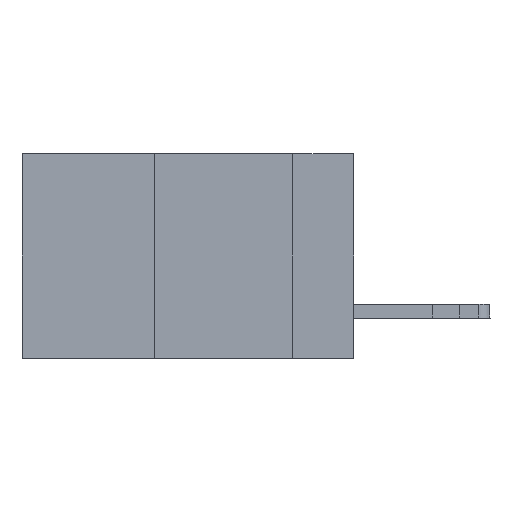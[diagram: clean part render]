
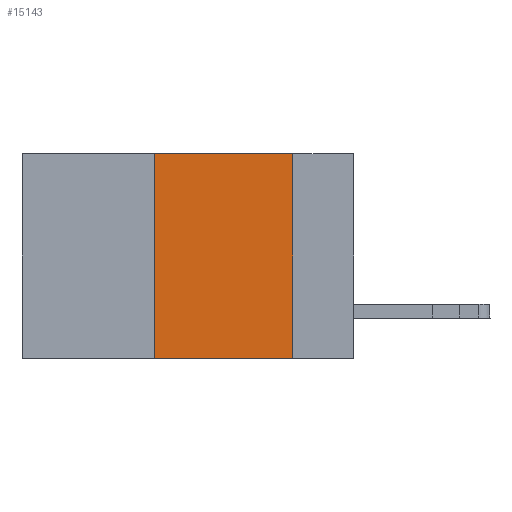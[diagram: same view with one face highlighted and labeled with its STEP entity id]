
A CAD part, left-side view. The second image highlights one B-rep face of the part: STEP entity #15143.
In plain terms, the highlighted planar face has unit normal (-1, 0, 0).
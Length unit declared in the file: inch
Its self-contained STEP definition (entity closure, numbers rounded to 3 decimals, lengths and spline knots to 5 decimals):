
#76 = DIRECTION ( 'NONE',  ( 0., -1., 0. ) ) ;
#1234 = ORIENTED_EDGE ( 'NONE', *, *, #23813, .F. ) ;
#3835 = CARTESIAN_POINT ( 'NONE',  ( 0., 0.6, 0. ) ) ;
#4667 = DIRECTION ( 'NONE',  ( 1., 0., 0. ) ) ;
#5010 = EDGE_CURVE ( 'NONE', #21064, #9253, #13825, .T. ) ;
#5304 = VERTEX_POINT ( 'NONE', #12621 ) ;
#5528 = LINE ( 'NONE', #25120, #19961 ) ;
#6491 = ORIENTED_EDGE ( 'NONE', *, *, #9548, .F. ) ;
#8597 = VECTOR ( 'NONE', #76, 39.37008 ) ;
#8794 = EDGE_LOOP ( 'NONE', ( #1234, #21076, #6491, #24580 ) ) ;
#9253 = VERTEX_POINT ( 'NONE', #19338 ) ;
#9548 = EDGE_CURVE ( 'NONE', #13042, #21064, #21270, .T. ) ;
#11204 = EDGE_CURVE ( 'NONE', #13042, #5304, #11600, .T. ) ;
#11600 = LINE ( 'NONE', #24869, #24228 ) ;
#12329 = CARTESIAN_POINT ( 'NONE',  ( 0., 0.36, 0. ) ) ;
#12369 = PLANE ( 'NONE',  #20666 ) ;
#12621 = CARTESIAN_POINT ( 'NONE',  ( 0., 0.11, -0.37 ) ) ;
#12717 = CARTESIAN_POINT ( 'NONE',  ( 0., 0.6, 0. ) ) ;
#13042 = VERTEX_POINT ( 'NONE', #22119 ) ;
#13337 = DIRECTION ( 'NONE',  ( 0., 0., -1. ) ) ;
#13752 = FACE_OUTER_BOUND ( 'NONE', #8794, .T. ) ;
#13825 = LINE ( 'NONE', #3835, #8597 ) ;
#15143 = ADVANCED_FACE ( 'NONE', ( #13752 ), #12369, .F. ) ;
#15992 = VECTOR ( 'NONE', #24594, 39.37008 ) ;
#18402 = DIRECTION ( 'NONE',  ( 0., 0., -1. ) ) ;
#19338 = CARTESIAN_POINT ( 'NONE',  ( 0., 0.11, 0. ) ) ;
#19961 = VECTOR ( 'NONE', #13337, 39.37008 ) ;
#19992 = CARTESIAN_POINT ( 'NONE',  ( 0., 0.36, 0. ) ) ;
#20666 = AXIS2_PLACEMENT_3D ( 'NONE', #12717, #4667, #18402 ) ;
#21012 = DIRECTION ( 'NONE',  ( 0., -1., 0. ) ) ;
#21064 = VERTEX_POINT ( 'NONE', #19992 ) ;
#21076 = ORIENTED_EDGE ( 'NONE', *, *, #5010, .F. ) ;
#21270 = LINE ( 'NONE', #12329, #15992 ) ;
#22119 = CARTESIAN_POINT ( 'NONE',  ( 0., 0.36, -0.37 ) ) ;
#23813 = EDGE_CURVE ( 'NONE', #9253, #5304, #5528, .T. ) ;
#24228 = VECTOR ( 'NONE', #21012, 39.37008 ) ;
#24580 = ORIENTED_EDGE ( 'NONE', *, *, #11204, .T. ) ;
#24594 = DIRECTION ( 'NONE',  ( 0., 0., 1. ) ) ;
#24869 = CARTESIAN_POINT ( 'NONE',  ( 0., 0.6, -0.37 ) ) ;
#25120 = CARTESIAN_POINT ( 'NONE',  ( 0., 0.11, 0. ) ) ;
